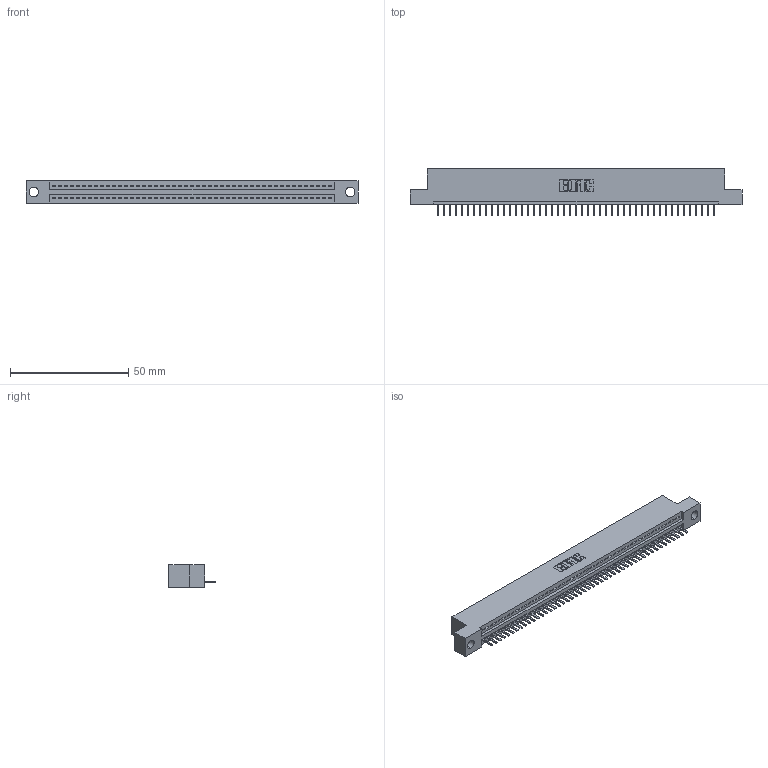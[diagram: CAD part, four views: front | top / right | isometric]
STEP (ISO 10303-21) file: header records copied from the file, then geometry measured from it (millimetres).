
FILE_DESCRIPTION (( 'STEP AP203' ), '1' );
FILE_NAME ('345-047-520-104.STEP', '2021-05-26T15:12:45', ( '' ), ( '' ), 'SwSTEP 2.0', 'SolidWorks 2020', '' );
FILE_SCHEMA (( 'CONFIG_CONTROL_DESIGN' ));
Length unit declared in the file: inch
Products named in the file (3): 345 Part_Flush Mounting Lugs - 0.156 Dia-TI; 345-047-520-104; 345-292-001_345-293-120
Assembly tree (48 placements, depth 2):
  345-047-520-104
    345 Part_Flush Mounting Lugs - 0.156 Dia-TI
    345-292-001_345-293-120  x47
Bounding box: 140.59 x 19.68 x 9.4 mm (x, y, z)
Volume: 13153.1 mm3; surface area: 16947.4 mm2
Topology: 48 solids, 48 shells, 3054 faces, 9025 edges, 5890 vertices
Faces by surface type: plane 2068, cylinder 986
Entity records: 35233 total; most frequent: CARTESIAN_POINT 6123, ORIENTED_EDGE 6090, DIRECTION 5327, EDGE_CURVE 3045, LINE 2721, VECTOR 2721, VERTEX_POINT 2026, AXIS2_PLACEMENT_3D 1303
